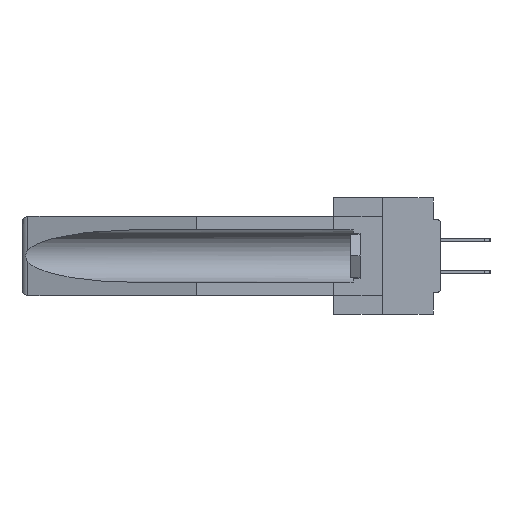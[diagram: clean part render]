
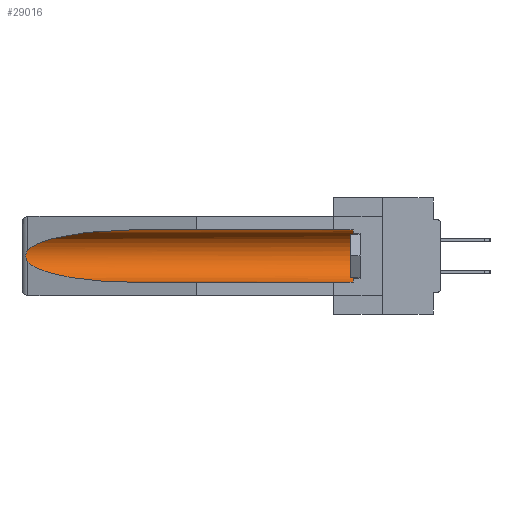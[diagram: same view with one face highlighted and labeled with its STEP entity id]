
A CAD part, left-side view. The second image highlights one B-rep face of the part: STEP entity #29016.
In plain terms, the highlighted cylindrical face has radius 2.857 mm (diameter 5.715 mm), a partial arc.
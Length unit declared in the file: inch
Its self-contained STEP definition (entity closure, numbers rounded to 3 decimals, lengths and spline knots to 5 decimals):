
#1215 = ORIENTED_EDGE ( 'NONE', *, *, #29212, .T. ) ;
#1968 = ORIENTED_EDGE ( 'NONE', *, *, #21923, .F. ) ;
#2149 = VECTOR ( 'NONE', #22032, 39.37008 ) ;
#2219 = LINE ( 'NONE', #12456, #2732 ) ;
#2372 = VERTEX_POINT ( 'NONE', #32876 ) ;
#2732 = VECTOR ( 'NONE', #15847, 39.37008 ) ;
#3059 = EDGE_LOOP ( 'NONE', ( #37544, #12829, #21561, #1968, #38796, #1215 ) ) ;
#5750 = CARTESIAN_POINT ( 'NONE',  ( 0.155, 0.126, -0.1715 ) ) ;
#6343 = CARTESIAN_POINT ( 'NONE',  ( 0.21114, 1.30732, -0.284 ) ) ;
#7861 = CARTESIAN_POINT ( 'NONE',  ( 0.21114, 1.30732, -0.059 ) ) ;
#8193 = EDGE_CURVE ( 'NONE', #15487, #21861, #26759, .T. ) ;
#9456 = CARTESIAN_POINT ( 'NONE',  ( 0.26537, 1.52718, -0.19328 ) ) ;
#9553 = CARTESIAN_POINT ( 'NONE',  ( 0.155, 1.07973, -0.059 ) ) ;
#9915 = CARTESIAN_POINT ( 'NONE',  ( 0.26655, 1.53094, -0.18657 ) ) ;
#10872 = CARTESIAN_POINT ( 'NONE',  ( 0.25451, 1.48313, -0.09465 ) ) ;
#11264 = LINE ( 'NONE', #42703, #2149 ) ;
#12456 = CARTESIAN_POINT ( 'NONE',  ( 0.155, -0.30754, -0.284 ) ) ;
#12829 = ORIENTED_EDGE ( 'NONE', *, *, #29992, .T. ) ;
#14397 = CIRCLE ( 'NONE', #24965, 0.1125 ) ;
#15487 = VERTEX_POINT ( 'NONE', #9553 ) ;
#15630 =( BOUNDED_CURVE ( )  B_SPLINE_CURVE ( 3, ( #33416, #37259, #6343, #17044 ),
 .UNSPECIFIED., .F., .F. ) 
 B_SPLINE_CURVE_WITH_KNOTS ( ( 4, 4 ),
 ( 0.1948, 1.5708 ),
 .UNSPECIFIED. ) 
 CURVE ( )  GEOMETRIC_REPRESENTATION_ITEM ( )  RATIONAL_B_SPLINE_CURVE ( ( 1., 0.848, 0.848, 1. ) ) 
 REPRESENTATION_ITEM ( '' )  );
#15847 = DIRECTION ( 'NONE',  ( 0., 1., 0. ) ) ;
#16017 = DIRECTION ( 'NONE',  ( 0., -1., 0. ) ) ;
#17044 = CARTESIAN_POINT ( 'NONE',  ( 0.155, 1.07973, -0.284 ) ) ;
#17474 = DIRECTION ( 'NONE',  ( 0., 1., 0. ) ) ;
#17772 = CARTESIAN_POINT ( 'NONE',  ( 0.155, -0.30754, -0.1715 ) ) ;
#19513 = CARTESIAN_POINT ( 'NONE',  ( 0.26597, 1.5296, -0.19026 ) ) ;
#19956 = CARTESIAN_POINT ( 'NONE',  ( 0.26654, 1.53092, -0.15636 ) ) ;
#20326 = CARTESIAN_POINT ( 'NONE',  ( 0.155, 0.126, -0.059 ) ) ;
#21561 = ORIENTED_EDGE ( 'NONE', *, *, #23898, .T. ) ;
#21785 = VERTEX_POINT ( 'NONE', #42587 ) ;
#21861 = VERTEX_POINT ( 'NONE', #36199 ) ;
#21923 = EDGE_CURVE ( 'NONE', #21785, #2372, #2219, .T. ) ;
#22032 = DIRECTION ( 'NONE',  ( 0., 1., 0. ) ) ;
#22342 = CYLINDRICAL_SURFACE ( 'NONE', #34003, 0.1125 ) ;
#23095 = DIRECTION ( 'NONE',  ( 0., 0., 1. ) ) ;
#23898 = EDGE_CURVE ( 'NONE', #24213, #2372, #15630, .T. ) ;
#24213 = VERTEX_POINT ( 'NONE', #31459 ) ;
#24577 = CARTESIAN_POINT ( 'NONE',  ( 0.155, 1.07973, -0.059 ) ) ;
#24841 = B_SPLINE_CURVE_WITH_KNOTS ( 'NONE', 3,
 ( #28989, #29142, #19956, #26315, #29560, #43011, #43466, #9915, #19513, #9456 ),
 .UNSPECIFIED., .F., .F.,
 ( 4, 2, 2, 2, 4 ),
 ( 0., 0.00029, 0.00058, 0.00087, 0.00117 ),
 .UNSPECIFIED. ) ;
#24965 = AXIS2_PLACEMENT_3D ( 'NONE', #5750, #16017, #23095 ) ;
#26315 = CARTESIAN_POINT ( 'NONE',  ( 0.2673, 1.5327, -0.16383 ) ) ;
#26759 =( BOUNDED_CURVE ( )  B_SPLINE_CURVE ( 3, ( #24577, #7861, #10872, #31492 ),
 .UNSPECIFIED., .F., .F. ) 
 B_SPLINE_CURVE_WITH_KNOTS ( ( 4, 4 ),
 ( 4.71239, 6.08839 ),
 .UNSPECIFIED. ) 
 CURVE ( )  GEOMETRIC_REPRESENTATION_ITEM ( )  RATIONAL_B_SPLINE_CURVE ( ( 1., 0.848, 0.848, 1. ) ) 
 REPRESENTATION_ITEM ( '' )  );
#28836 = EDGE_CURVE ( 'NONE', #21785, #31486, #14397, .T. ) ;
#28989 = CARTESIAN_POINT ( 'NONE',  ( 0.26537, 1.52718, -0.14972 ) ) ;
#29016 = ADVANCED_FACE ( 'NONE', ( #29237 ), #22342, .F. ) ;
#29142 = CARTESIAN_POINT ( 'NONE',  ( 0.26597, 1.52961, -0.15275 ) ) ;
#29212 = EDGE_CURVE ( 'NONE', #31486, #15487, #11264, .T. ) ;
#29237 = FACE_OUTER_BOUND ( 'NONE', #3059, .T. ) ;
#29560 = CARTESIAN_POINT ( 'NONE',  ( 0.2675, 1.53308, -0.16763 ) ) ;
#29992 = EDGE_CURVE ( 'NONE', #21861, #24213, #24841, .T. ) ;
#31459 = CARTESIAN_POINT ( 'NONE',  ( 0.26537, 1.52718, -0.19328 ) ) ;
#31486 = VERTEX_POINT ( 'NONE', #20326 ) ;
#31492 = CARTESIAN_POINT ( 'NONE',  ( 0.26537, 1.52718, -0.14972 ) ) ;
#32876 = CARTESIAN_POINT ( 'NONE',  ( 0.155, 1.07973, -0.284 ) ) ;
#33416 = CARTESIAN_POINT ( 'NONE',  ( 0.26537, 1.52718, -0.19328 ) ) ;
#34003 = AXIS2_PLACEMENT_3D ( 'NONE', #17772, #17474, #37412 ) ;
#36199 = CARTESIAN_POINT ( 'NONE',  ( 0.26537, 1.52718, -0.14972 ) ) ;
#37259 = CARTESIAN_POINT ( 'NONE',  ( 0.25451, 1.48313, -0.24835 ) ) ;
#37412 = DIRECTION ( 'NONE',  ( 0., 0., 1. ) ) ;
#37544 = ORIENTED_EDGE ( 'NONE', *, *, #8193, .T. ) ;
#38796 = ORIENTED_EDGE ( 'NONE', *, *, #28836, .T. ) ;
#42587 = CARTESIAN_POINT ( 'NONE',  ( 0.155, 0.126, -0.284 ) ) ;
#42703 = CARTESIAN_POINT ( 'NONE',  ( 0.155, -0.30754, -0.059 ) ) ;
#43011 = CARTESIAN_POINT ( 'NONE',  ( 0.2675, 1.53308, -0.17534 ) ) ;
#43466 = CARTESIAN_POINT ( 'NONE',  ( 0.2673, 1.53269, -0.17917 ) ) ;
